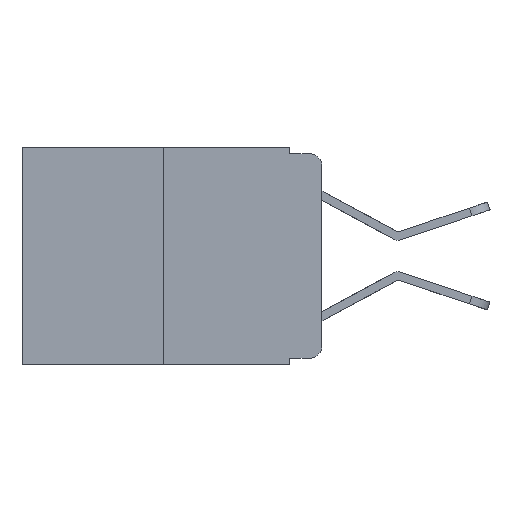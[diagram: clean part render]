
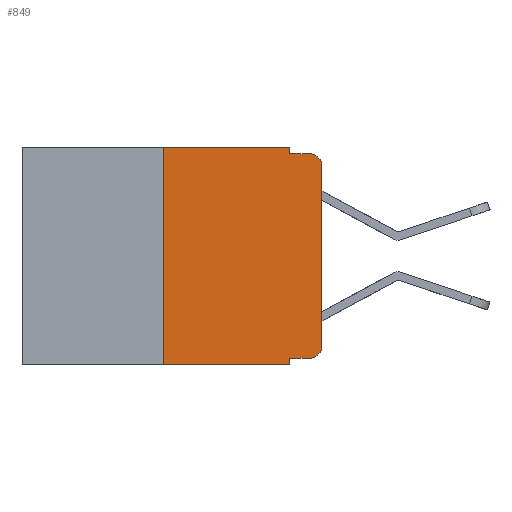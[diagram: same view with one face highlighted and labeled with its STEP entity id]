
A CAD part, left-side view. The second image highlights one B-rep face of the part: STEP entity #849.
In plain terms, the highlighted planar face has unit normal (-1, 0, 0).
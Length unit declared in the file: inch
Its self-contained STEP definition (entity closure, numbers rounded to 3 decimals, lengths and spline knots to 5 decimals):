
#77 = LINE ( 'NONE', #21204, #13630 ) ;
#299 = ORIENTED_EDGE ( 'NONE', *, *, #15182, .F. ) ;
#337 = CARTESIAN_POINT ( 'NONE',  ( 0., 0.051, 0. ) ) ;
#410 = AXIS2_PLACEMENT_3D ( 'NONE', #19760, #9397, #21438 ) ;
#648 = ORIENTED_EDGE ( 'NONE', *, *, #5304, .T. ) ;
#770 = CARTESIAN_POINT ( 'NONE',  ( 0., 0.02, -0.03 ) ) ;
#824 = AXIS2_PLACEMENT_3D ( 'NONE', #770, #13132, #2588 ) ;
#849 = ADVANCED_FACE ( 'NONE', ( #11934 ), #16626, .F. ) ;
#1553 = EDGE_CURVE ( 'NONE', #20454, #11718, #5839, .T. ) ;
#1634 = ORIENTED_EDGE ( 'NONE', *, *, #4786, .T. ) ;
#1965 = CARTESIAN_POINT ( 'NONE',  ( 0., 0.051, -0.01 ) ) ;
#2015 = ORIENTED_EDGE ( 'NONE', *, *, #4050, .T. ) ;
#2272 = EDGE_CURVE ( 'NONE', #18867, #10862, #6092, .T. ) ;
#2588 = DIRECTION ( 'NONE',  ( 0., 0., -1. ) ) ;
#3284 = LINE ( 'NONE', #16830, #15562 ) ;
#3651 = EDGE_CURVE ( 'NONE', #7579, #18867, #3284, .T. ) ;
#4017 = VERTEX_POINT ( 'NONE', #11478 ) ;
#4050 = EDGE_CURVE ( 'NONE', #4017, #11590, #7683, .T. ) ;
#4786 = EDGE_CURVE ( 'NONE', #11590, #20887, #6256, .T. ) ;
#5187 = DIRECTION ( 'NONE',  ( 0., -1., 0. ) ) ;
#5304 = EDGE_CURVE ( 'NONE', #20887, #19584, #77, .T. ) ;
#5312 = VERTEX_POINT ( 'NONE', #5665 ) ;
#5665 = CARTESIAN_POINT ( 'NONE',  ( 0., 0.02, -0.01 ) ) ;
#5839 = LINE ( 'NONE', #20375, #10514 ) ;
#6092 = LINE ( 'NONE', #19283, #14782 ) ;
#6256 = CIRCLE ( 'NONE', #410, 0.02 ) ;
#6648 = EDGE_CURVE ( 'NONE', #4017, #11718, #11714, .T. ) ;
#7405 = CARTESIAN_POINT ( 'NONE',  ( 0., 0.473, 0. ) ) ;
#7532 = ORIENTED_EDGE ( 'NONE', *, *, #19857, .F. ) ;
#7579 = VERTEX_POINT ( 'NONE', #13707 ) ;
#7683 = LINE ( 'NONE', #7933, #15802 ) ;
#7789 = VECTOR ( 'NONE', #5187, 39.37008 ) ;
#7933 = CARTESIAN_POINT ( 'NONE',  ( 0., 0.051, -0.333 ) ) ;
#7973 = DIRECTION ( 'NONE',  ( 0., -1., 0. ) ) ;
#8014 = CARTESIAN_POINT ( 'NONE',  ( 0., 0.25, -0.343 ) ) ;
#9240 = DIRECTION ( 'NONE',  ( 0., 0., -1. ) ) ;
#9346 = ORIENTED_EDGE ( 'NONE', *, *, #1553, .T. ) ;
#9397 = DIRECTION ( 'NONE',  ( -1., 0., 0. ) ) ;
#9778 = CARTESIAN_POINT ( 'NONE',  ( 0., 0.051, -0.343 ) ) ;
#10514 = VECTOR ( 'NONE', #7973, 39.37008 ) ;
#10862 = VERTEX_POINT ( 'NONE', #1965 ) ;
#11430 = DIRECTION ( 'NONE',  ( 0., -1., 0. ) ) ;
#11478 = CARTESIAN_POINT ( 'NONE',  ( 0., 0.051, -0.333 ) ) ;
#11590 = VERTEX_POINT ( 'NONE', #12612 ) ;
#11714 = LINE ( 'NONE', #337, #15163 ) ;
#11718 = VERTEX_POINT ( 'NONE', #9778 ) ;
#11934 = FACE_OUTER_BOUND ( 'NONE', #11994, .T. ) ;
#11994 = EDGE_LOOP ( 'NONE', ( #648, #18768, #299, #15250, #16819, #7532, #9346, #19441, #2015, #1634 ) ) ;
#12110 = AXIS2_PLACEMENT_3D ( 'NONE', #7405, #19125, #18962 ) ;
#12612 = CARTESIAN_POINT ( 'NONE',  ( 0., 0.02, -0.333 ) ) ;
#12792 = CARTESIAN_POINT ( 'NONE',  ( 0., 0., -0.313 ) ) ;
#13132 = DIRECTION ( 'NONE',  ( -1., 0., 0. ) ) ;
#13630 = VECTOR ( 'NONE', #19519, 39.37008 ) ;
#13707 = CARTESIAN_POINT ( 'NONE',  ( 0., 0.25, 0. ) ) ;
#13893 = CARTESIAN_POINT ( 'NONE',  ( 0., 0.051, -0.01 ) ) ;
#14039 = CARTESIAN_POINT ( 'NONE',  ( 0., 0.051, 0. ) ) ;
#14678 = VECTOR ( 'NONE', #15128, 39.37008 ) ;
#14782 = VECTOR ( 'NONE', #17760, 39.37008 ) ;
#15009 = DIRECTION ( 'NONE',  ( 0., -1., 0. ) ) ;
#15128 = DIRECTION ( 'NONE',  ( 0., 0., 1. ) ) ;
#15163 = VECTOR ( 'NONE', #9240, 39.37008 ) ;
#15182 = EDGE_CURVE ( 'NONE', #10862, #5312, #21028, .T. ) ;
#15250 = ORIENTED_EDGE ( 'NONE', *, *, #2272, .F. ) ;
#15562 = VECTOR ( 'NONE', #15009, 39.37008 ) ;
#15802 = VECTOR ( 'NONE', #11430, 39.37008 ) ;
#15984 = CARTESIAN_POINT ( 'NONE',  ( 0., 0., -0.03 ) ) ;
#16568 = EDGE_CURVE ( 'NONE', #19584, #5312, #19212, .T. ) ;
#16626 = PLANE ( 'NONE',  #12110 ) ;
#16819 = ORIENTED_EDGE ( 'NONE', *, *, #3651, .F. ) ;
#16830 = CARTESIAN_POINT ( 'NONE',  ( 0., 0.473, 0. ) ) ;
#17760 = DIRECTION ( 'NONE',  ( 0., 0., -1. ) ) ;
#18587 = CARTESIAN_POINT ( 'NONE',  ( 0., 0.25, 0. ) ) ;
#18768 = ORIENTED_EDGE ( 'NONE', *, *, #16568, .T. ) ;
#18867 = VERTEX_POINT ( 'NONE', #14039 ) ;
#18962 = DIRECTION ( 'NONE',  ( 0., 0., -1. ) ) ;
#19125 = DIRECTION ( 'NONE',  ( 1., 0., 0. ) ) ;
#19212 = CIRCLE ( 'NONE', #824, 0.02 ) ;
#19283 = CARTESIAN_POINT ( 'NONE',  ( 0., 0.051, 0. ) ) ;
#19327 = LINE ( 'NONE', #18587, #14678 ) ;
#19441 = ORIENTED_EDGE ( 'NONE', *, *, #6648, .F. ) ;
#19519 = DIRECTION ( 'NONE',  ( 0., 0., 1. ) ) ;
#19584 = VERTEX_POINT ( 'NONE', #15984 ) ;
#19760 = CARTESIAN_POINT ( 'NONE',  ( 0., 0.02, -0.313 ) ) ;
#19857 = EDGE_CURVE ( 'NONE', #20454, #7579, #19327, .T. ) ;
#20375 = CARTESIAN_POINT ( 'NONE',  ( 0., 0.473, -0.343 ) ) ;
#20454 = VERTEX_POINT ( 'NONE', #8014 ) ;
#20887 = VERTEX_POINT ( 'NONE', #12792 ) ;
#21028 = LINE ( 'NONE', #13893, #7789 ) ;
#21204 = CARTESIAN_POINT ( 'NONE',  ( 0., 0., 0. ) ) ;
#21438 = DIRECTION ( 'NONE',  ( 0., 0., -1. ) ) ;
